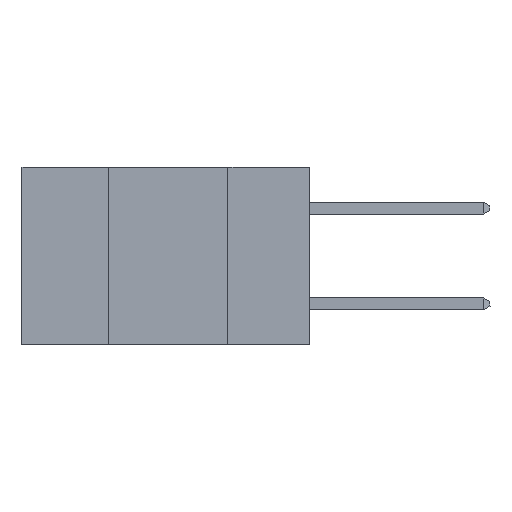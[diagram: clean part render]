
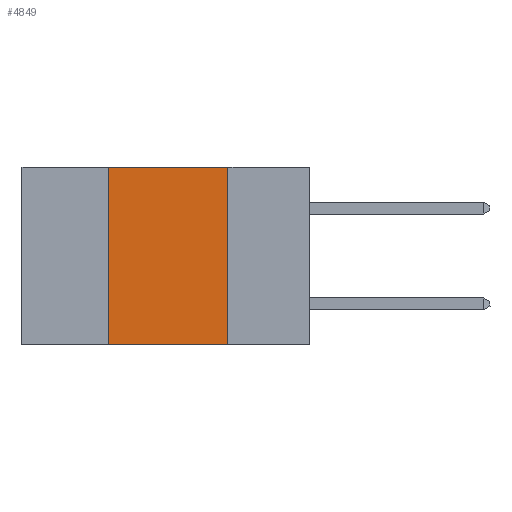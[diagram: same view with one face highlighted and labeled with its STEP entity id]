
A CAD part, left-side view. The second image highlights one B-rep face of the part: STEP entity #4849.
In plain terms, the highlighted planar face has unit normal (-1, 0, 0).
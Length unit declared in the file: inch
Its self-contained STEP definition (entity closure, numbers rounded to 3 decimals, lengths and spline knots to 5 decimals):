
#302 = VECTOR ( 'NONE', #2837, 39.37008 ) ;
#417 = VECTOR ( 'NONE', #13007, 39.37008 ) ;
#1273 = CARTESIAN_POINT ( 'NONE',  ( 0., 0.17, 0. ) ) ;
#2689 = AXIS2_PLACEMENT_3D ( 'NONE', #11153, #14279, #4890 ) ;
#2752 = ORIENTED_EDGE ( 'NONE', *, *, #16773, .F. ) ;
#2837 = DIRECTION ( 'NONE',  ( 0., -1., 0. ) ) ;
#3071 = VERTEX_POINT ( 'NONE', #13852 ) ;
#3584 = ORIENTED_EDGE ( 'NONE', *, *, #18567, .F. ) ;
#3586 = CARTESIAN_POINT ( 'NONE',  ( 0., 0.6, -0.37 ) ) ;
#3811 = ORIENTED_EDGE ( 'NONE', *, *, #13521, .T. ) ;
#4849 = ADVANCED_FACE ( 'NONE', ( #10643 ), #9605, .F. ) ;
#4890 = DIRECTION ( 'NONE',  ( 0., 0., -1. ) ) ;
#5027 = LINE ( 'NONE', #10677, #302 ) ;
#8336 = LINE ( 'NONE', #8841, #12970 ) ;
#8378 = LINE ( 'NONE', #3586, #417 ) ;
#8380 = EDGE_LOOP ( 'NONE', ( #8768, #2752, #3584, #3811 ) ) ;
#8768 = ORIENTED_EDGE ( 'NONE', *, *, #10755, .F. ) ;
#8841 = CARTESIAN_POINT ( 'NONE',  ( 0., 0.17, 0. ) ) ;
#9302 = DIRECTION ( 'NONE',  ( 0., 0., 1. ) ) ;
#9605 = PLANE ( 'NONE',  #2689 ) ;
#10643 = FACE_OUTER_BOUND ( 'NONE', #8380, .T. ) ;
#10677 = CARTESIAN_POINT ( 'NONE',  ( 0., 0.6, 0. ) ) ;
#10755 = EDGE_CURVE ( 'NONE', #19168, #16571, #8336, .T. ) ;
#11153 = CARTESIAN_POINT ( 'NONE',  ( 0., 0.6, 0. ) ) ;
#11797 = CARTESIAN_POINT ( 'NONE',  ( 0., 0.42, -0.37 ) ) ;
#12970 = VECTOR ( 'NONE', #19510, 39.37008 ) ;
#13007 = DIRECTION ( 'NONE',  ( 0., -1., 0. ) ) ;
#13521 = EDGE_CURVE ( 'NONE', #14868, #16571, #8378, .T. ) ;
#13852 = CARTESIAN_POINT ( 'NONE',  ( 0., 0.42, 0. ) ) ;
#14279 = DIRECTION ( 'NONE',  ( 1., 0., 0. ) ) ;
#14820 = LINE ( 'NONE', #18349, #18338 ) ;
#14868 = VERTEX_POINT ( 'NONE', #11797 ) ;
#16571 = VERTEX_POINT ( 'NONE', #17907 ) ;
#16773 = EDGE_CURVE ( 'NONE', #3071, #19168, #5027, .T. ) ;
#17907 = CARTESIAN_POINT ( 'NONE',  ( 0., 0.17, -0.37 ) ) ;
#18338 = VECTOR ( 'NONE', #9302, 39.37008 ) ;
#18349 = CARTESIAN_POINT ( 'NONE',  ( 0., 0.42, 0. ) ) ;
#18567 = EDGE_CURVE ( 'NONE', #14868, #3071, #14820, .T. ) ;
#19168 = VERTEX_POINT ( 'NONE', #1273 ) ;
#19510 = DIRECTION ( 'NONE',  ( 0., 0., -1. ) ) ;
